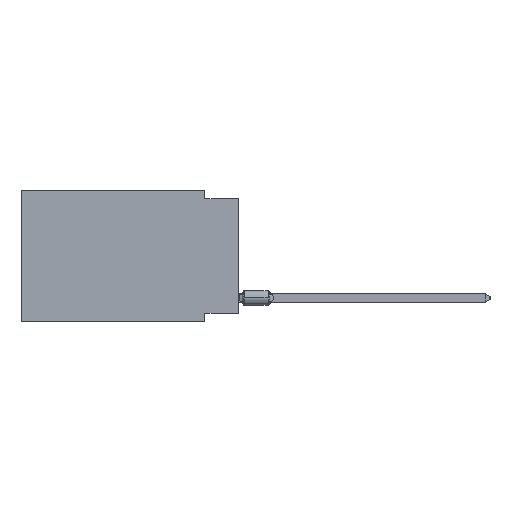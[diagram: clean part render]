
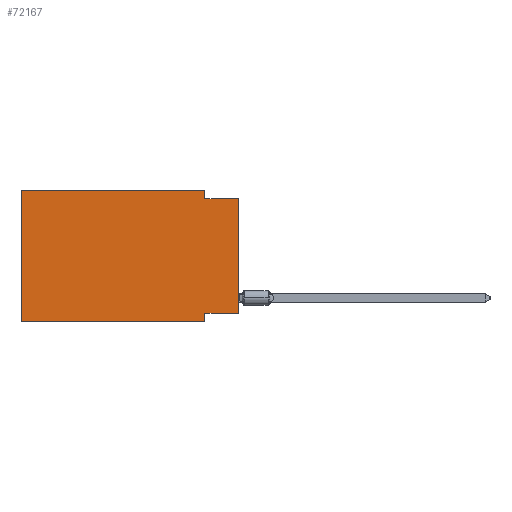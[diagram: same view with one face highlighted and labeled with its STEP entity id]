
A CAD part, left-side view. The second image highlights one B-rep face of the part: STEP entity #72167.
In plain terms, the highlighted planar face has unit normal (-1, 0, 0).
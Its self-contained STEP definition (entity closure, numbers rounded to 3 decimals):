
#414 = VECTOR ( 'NONE', #19776, 1000. ) ;
#2459 = EDGE_CURVE ( 'NONE', #54489, #32367, #12754, .T. ) ;
#3494 = VECTOR ( 'NONE', #57112, 1000. ) ;
#5434 = VECTOR ( 'NONE', #58552, 1000. ) ;
#5880 = VECTOR ( 'NONE', #69143, 1000. ) ;
#7162 = EDGE_CURVE ( 'NONE', #30141, #54489, #25787, .T. ) ;
#7682 = LINE ( 'NONE', #37391, #59309 ) ;
#9602 = VECTOR ( 'NONE', #35692, 1000. ) ;
#9630 = VERTEX_POINT ( 'NONE', #53139 ) ;
#10191 = CARTESIAN_POINT ( 'NONE',  ( 0., 2.54, -9.906 ) ) ;
#10937 = LINE ( 'NONE', #10191, #54666 ) ;
#11097 = EDGE_CURVE ( 'NONE', #41996, #34196, #63443, .T. ) ;
#11617 = CARTESIAN_POINT ( 'NONE',  ( 0., 2.54, 0. ) ) ;
#12754 = LINE ( 'NONE', #23639, #9602 ) ;
#13379 = CARTESIAN_POINT ( 'NONE',  ( 0., 2.54, -9.906 ) ) ;
#13926 = PLANE ( 'NONE',  #71229 ) ;
#17717 = EDGE_CURVE ( 'NONE', #41996, #59027, #40556, .T. ) ;
#19776 = DIRECTION ( 'NONE',  ( 0., 0., -1. ) ) ;
#21076 = CARTESIAN_POINT ( 'NONE',  ( 0., 2.54, -0.635 ) ) ;
#21105 = DIRECTION ( 'NONE',  ( 0., 0., -1. ) ) ;
#23040 = CARTESIAN_POINT ( 'NONE',  ( 0., 0., -9.271 ) ) ;
#23357 = CARTESIAN_POINT ( 'NONE',  ( 0., 16.383, 0. ) ) ;
#23461 = EDGE_CURVE ( 'NONE', #56984, #32367, #7682, .T. ) ;
#23639 = CARTESIAN_POINT ( 'NONE',  ( 0., 0., -0.635 ) ) ;
#24342 = CARTESIAN_POINT ( 'NONE',  ( 0., 0., -0.635 ) ) ;
#25787 = LINE ( 'NONE', #71715, #414 ) ;
#26913 = CARTESIAN_POINT ( 'NONE',  ( 0., 16.383, 0. ) ) ;
#27908 = DIRECTION ( 'NONE',  ( 0., -1., 0. ) ) ;
#27929 = EDGE_LOOP ( 'NONE', ( #32061, #61035, #31615, #52669, #43388, #36740, #65415, #52638 ) ) ;
#30141 = VERTEX_POINT ( 'NONE', #11617 ) ;
#31615 = ORIENTED_EDGE ( 'NONE', *, *, #7162, .F. ) ;
#31957 = FACE_OUTER_BOUND ( 'NONE', #27929, .T. ) ;
#32061 = ORIENTED_EDGE ( 'NONE', *, *, #23461, .T. ) ;
#32367 = VERTEX_POINT ( 'NONE', #24342 ) ;
#33285 = VECTOR ( 'NONE', #27908, 1000. ) ;
#34196 = VERTEX_POINT ( 'NONE', #13379 ) ;
#35610 = CARTESIAN_POINT ( 'NONE',  ( 0., 16.383, -9.906 ) ) ;
#35692 = DIRECTION ( 'NONE',  ( 0., -1., 0. ) ) ;
#36740 = ORIENTED_EDGE ( 'NONE', *, *, #11097, .T. ) ;
#37391 = CARTESIAN_POINT ( 'NONE',  ( 0., 0., 0. ) ) ;
#40556 = LINE ( 'NONE', #56748, #3494 ) ;
#41996 = VERTEX_POINT ( 'NONE', #54067 ) ;
#43388 = ORIENTED_EDGE ( 'NONE', *, *, #17717, .F. ) ;
#48085 = EDGE_CURVE ( 'NONE', #56984, #9630, #69521, .T. ) ;
#51223 = LINE ( 'NONE', #23357, #33285 ) ;
#51746 = EDGE_CURVE ( 'NONE', #9630, #34196, #10937, .T. ) ;
#52638 = ORIENTED_EDGE ( 'NONE', *, *, #48085, .F. ) ;
#52669 = ORIENTED_EDGE ( 'NONE', *, *, #64344, .F. ) ;
#53139 = CARTESIAN_POINT ( 'NONE',  ( 0., 2.54, -9.271 ) ) ;
#54067 = CARTESIAN_POINT ( 'NONE',  ( 0., 16.383, -9.906 ) ) ;
#54489 = VERTEX_POINT ( 'NONE', #21076 ) ;
#54666 = VECTOR ( 'NONE', #21105, 1000. ) ;
#56748 = CARTESIAN_POINT ( 'NONE',  ( 0., 16.383, 0. ) ) ;
#56984 = VERTEX_POINT ( 'NONE', #23040 ) ;
#57112 = DIRECTION ( 'NONE',  ( 0., 0., 1. ) ) ;
#58552 = DIRECTION ( 'NONE',  ( 0., -1., 0. ) ) ;
#59027 = VERTEX_POINT ( 'NONE', #26913 ) ;
#59309 = VECTOR ( 'NONE', #71265, 1000. ) ;
#60550 = DIRECTION ( 'NONE',  ( 1., 0., 0. ) ) ;
#61035 = ORIENTED_EDGE ( 'NONE', *, *, #2459, .F. ) ;
#63443 = LINE ( 'NONE', #35610, #5434 ) ;
#64344 = EDGE_CURVE ( 'NONE', #59027, #30141, #51223, .T. ) ;
#65415 = ORIENTED_EDGE ( 'NONE', *, *, #51746, .F. ) ;
#66202 = DIRECTION ( 'NONE',  ( 0., 0., -1. ) ) ;
#69143 = DIRECTION ( 'NONE',  ( 0., 1., 0. ) ) ;
#69521 = LINE ( 'NONE', #69891, #5880 ) ;
#69891 = CARTESIAN_POINT ( 'NONE',  ( 0., 0., -9.271 ) ) ;
#71229 = AXIS2_PLACEMENT_3D ( 'NONE', #71475, #60550, #66202 ) ;
#71265 = DIRECTION ( 'NONE',  ( 0., 0., 1. ) ) ;
#71475 = CARTESIAN_POINT ( 'NONE',  ( 0., 16.383, 0. ) ) ;
#71715 = CARTESIAN_POINT ( 'NONE',  ( 0., 2.54, 0. ) ) ;
#72167 = ADVANCED_FACE ( 'NONE', ( #31957 ), #13926, .F. ) ;
